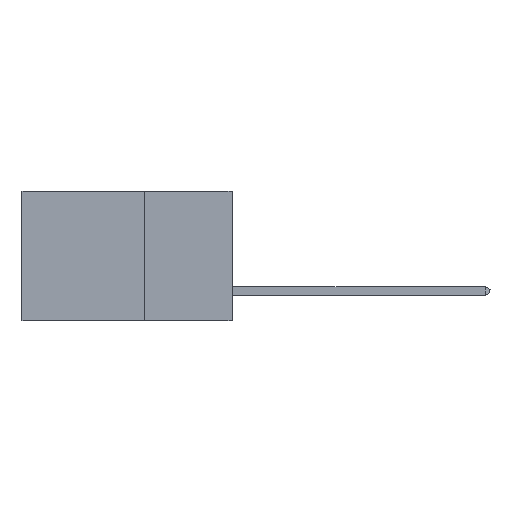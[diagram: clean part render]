
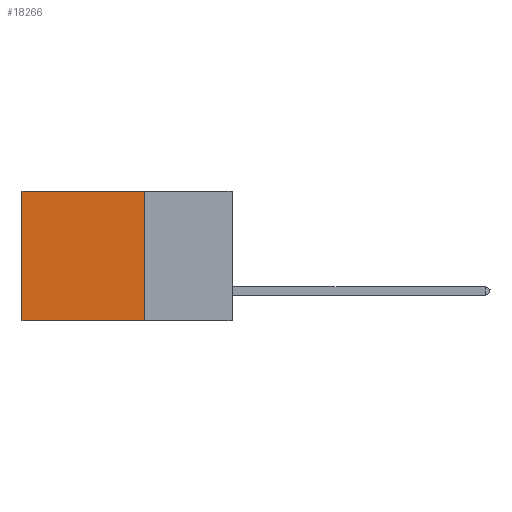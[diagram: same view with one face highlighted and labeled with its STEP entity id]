
A CAD part, left-side view. The second image highlights one B-rep face of the part: STEP entity #18266.
In plain terms, the highlighted planar face has unit normal (-1, 0, 0).
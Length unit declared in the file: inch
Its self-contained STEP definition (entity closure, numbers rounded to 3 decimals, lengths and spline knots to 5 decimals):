
#1083 = VECTOR ( 'NONE', #18948, 39.37008 ) ;
#2474 = CARTESIAN_POINT ( 'NONE',  ( 0.2875, 0.25, 0. ) ) ;
#2775 = CARTESIAN_POINT ( 'NONE',  ( 0.2875, 0.6, -0.37 ) ) ;
#5151 = DIRECTION ( 'NONE',  ( 1., 0., 0. ) ) ;
#5753 = DIRECTION ( 'NONE',  ( 0., 0., -1. ) ) ;
#6090 = DIRECTION ( 'NONE',  ( 0., 1., 0. ) ) ;
#6339 = CARTESIAN_POINT ( 'NONE',  ( 0.2875, 0.25, -0.37 ) ) ;
#8900 = VERTEX_POINT ( 'NONE', #2474 ) ;
#9161 = LINE ( 'NONE', #39548, #27840 ) ;
#11726 = VERTEX_POINT ( 'NONE', #19156 ) ;
#14603 = AXIS2_PLACEMENT_3D ( 'NONE', #46393, #5151, #31336 ) ;
#15189 = CARTESIAN_POINT ( 'NONE',  ( 0.2875, 0.25, -0.37 ) ) ;
#18030 = EDGE_CURVE ( 'NONE', #11726, #39583, #9161, .T. ) ;
#18200 = VERTEX_POINT ( 'NONE', #6339 ) ;
#18266 = ADVANCED_FACE ( 'NONE', ( #19037 ), #45743, .F. ) ;
#18948 = DIRECTION ( 'NONE',  ( 0., 1., 0. ) ) ;
#19037 = FACE_OUTER_BOUND ( 'NONE', #26322, .T. ) ;
#19156 = CARTESIAN_POINT ( 'NONE',  ( 0.2875, 0.6, 0. ) ) ;
#21256 = EDGE_CURVE ( 'NONE', #8900, #11726, #34955, .T. ) ;
#21972 = VECTOR ( 'NONE', #5753, 39.37008 ) ;
#26322 = EDGE_LOOP ( 'NONE', ( #28198, #33582, #32810, #36411 ) ) ;
#27618 = CARTESIAN_POINT ( 'NONE',  ( 0.2875, 0.25, 0. ) ) ;
#27840 = VECTOR ( 'NONE', #43312, 39.37008 ) ;
#28198 = ORIENTED_EDGE ( 'NONE', *, *, #18030, .T. ) ;
#28953 = LINE ( 'NONE', #27618, #21972 ) ;
#31336 = DIRECTION ( 'NONE',  ( 0., 0., -1. ) ) ;
#31773 = CARTESIAN_POINT ( 'NONE',  ( 0.2875, 0.25, 0. ) ) ;
#32642 = VECTOR ( 'NONE', #6090, 39.37008 ) ;
#32810 = ORIENTED_EDGE ( 'NONE', *, *, #44963, .F. ) ;
#33582 = ORIENTED_EDGE ( 'NONE', *, *, #38169, .F. ) ;
#34955 = LINE ( 'NONE', #31773, #32642 ) ;
#36411 = ORIENTED_EDGE ( 'NONE', *, *, #21256, .T. ) ;
#36455 = LINE ( 'NONE', #15189, #1083 ) ;
#38169 = EDGE_CURVE ( 'NONE', #18200, #39583, #36455, .T. ) ;
#39548 = CARTESIAN_POINT ( 'NONE',  ( 0.2875, 0.6, 0. ) ) ;
#39583 = VERTEX_POINT ( 'NONE', #2775 ) ;
#43312 = DIRECTION ( 'NONE',  ( 0., 0., -1. ) ) ;
#44963 = EDGE_CURVE ( 'NONE', #8900, #18200, #28953, .T. ) ;
#45743 = PLANE ( 'NONE',  #14603 ) ;
#46393 = CARTESIAN_POINT ( 'NONE',  ( 0.2875, 0.25, 0. ) ) ;
